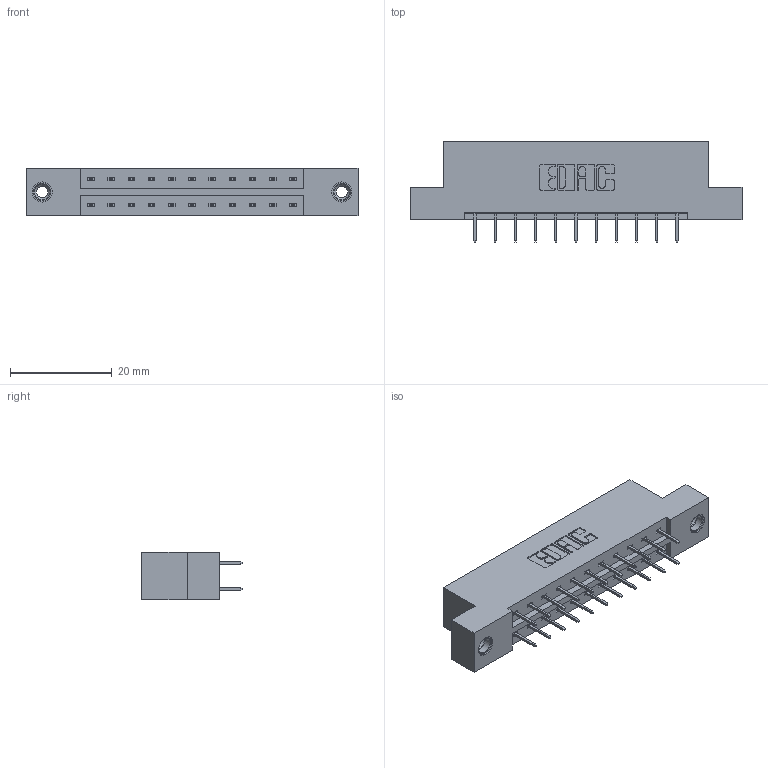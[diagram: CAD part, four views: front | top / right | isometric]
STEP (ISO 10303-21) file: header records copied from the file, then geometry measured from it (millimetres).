
FILE_DESCRIPTION (( 'STEP AP203' ), '1' );
FILE_NAME ('833-022-524-208.STEP', '2020-06-01T16:40:45', ( '' ), ( '' ), 'SwSTEP 2.0', 'SolidWorks 2020', '' );
FILE_SCHEMA (( 'CONFIG_CONTROL_DESIGN' ));
Length unit declared in the file: inch
Products named in the file (4): 833-022-524-208; 833 Part_Flush - .156 Dia - TI; 345-250-001_345-250-003-102; 345-292-001_345-293-124
Assembly tree (25 placements, depth 2):
  833-022-524-208
    833 Part_Flush - .156 Dia - TI
    345-292-001_345-293-124  x22
    345-250-001_345-250-003-102  x2
Bounding box: 65.13 x 19.69 x 9.4 mm (x, y, z)
Volume: 6319.2 mm3; surface area: 7059.6 mm2
Topology: 25 solids, 25 shells, 1406 faces, 3945 edges, 2534 vertices
Faces by surface type: plane 1026, cylinder 364, cone 12, torus 4
Entity records: 12346 total; most frequent: CARTESIAN_POINT 2065, ORIENTED_EDGE 1994, DIRECTION 1851, EDGE_CURVE 997, VECTOR 853, LINE 853, VERTEX_POINT 656, AXIS2_PLACEMENT_3D 499
